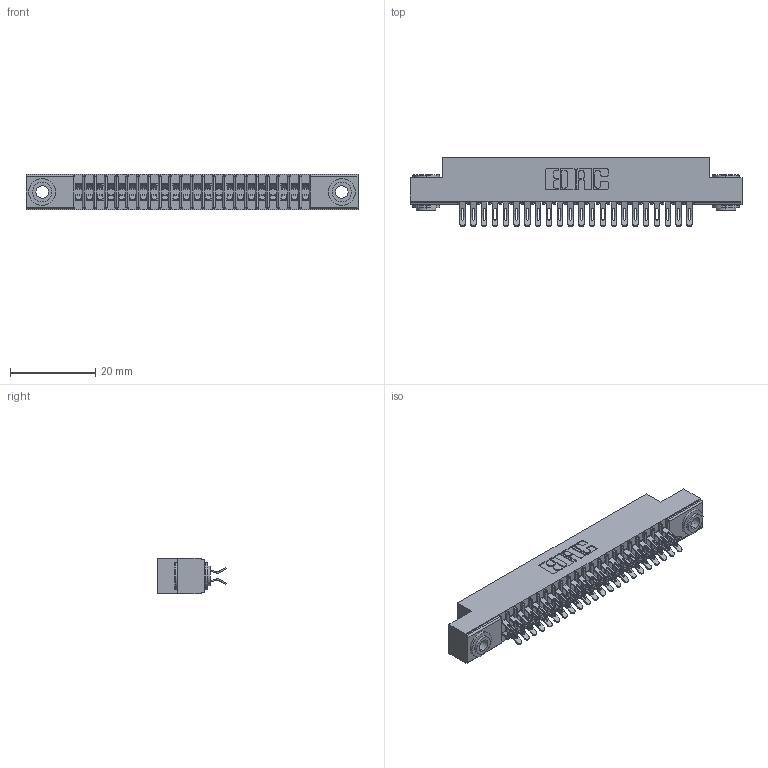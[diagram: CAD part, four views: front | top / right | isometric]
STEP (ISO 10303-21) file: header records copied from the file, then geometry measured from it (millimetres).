
FILE_DESCRIPTION (( 'STEP AP203' ), '1' );
FILE_NAME ('341-044-555-203.STEP', '2018-08-07T02:43:09', ( '' ), ( '' ), 'SwSTEP 2.0', 'SolidWorks 2016', '' );
FILE_SCHEMA (( 'CONFIG_CONTROL_DESIGN' ));
Length unit declared in the file: inch
Products named in the file (4): 341-292-001_341-292-155; 345-250-002_345-250-002-102; 341-044-555-203; 341 Part_.156 (3.96) Dia Mounting Holes
Assembly tree (47 placements, depth 2):
  341-044-555-203
    341 Part_.156 (3.96) Dia Mounting Holes
    341-292-001_341-292-155  x44
    345-250-002_345-250-002-102  x2
Bounding box: 78.11 x 16.31 x 8.38 mm (x, y, z)
Volume: 4503.8 mm3; surface area: 9966.1 mm2
Topology: 47 solids, 47 shells, 3600 faces, 10702 edges, 6966 vertices
Faces by surface type: plane 1940, cylinder 1564, sphere 46, torus 42, cone 8
Entity records: 30824 total; most frequent: CARTESIAN_POINT 5121, ORIENTED_EDGE 5068, DIRECTION 4990, EDGE_CURVE 2534, VECTOR 2000, LINE 2000, VERTEX_POINT 1610, AXIS2_PLACEMENT_3D 1495
